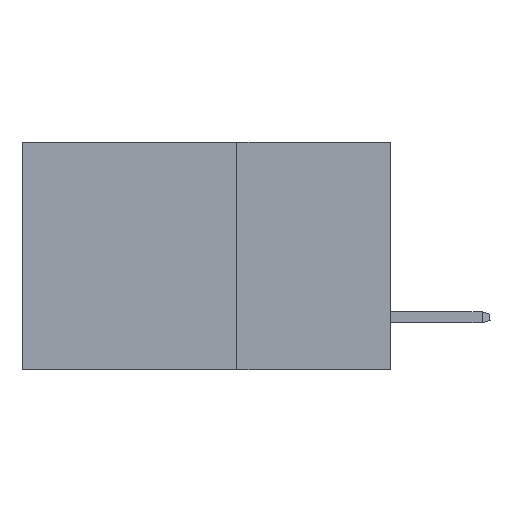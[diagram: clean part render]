
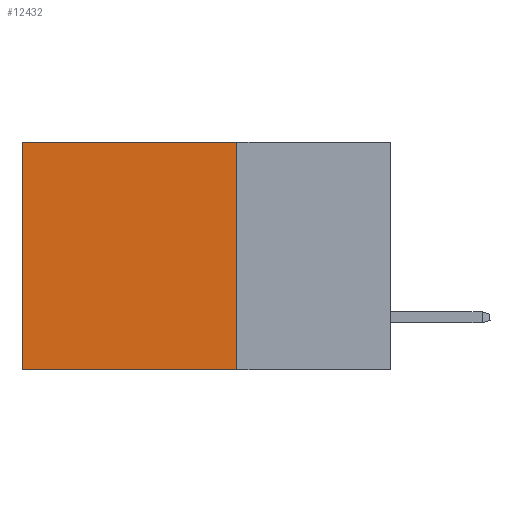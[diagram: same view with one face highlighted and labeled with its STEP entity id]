
A CAD part, left-side view. The second image highlights one B-rep face of the part: STEP entity #12432.
In plain terms, the highlighted planar face has unit normal (-1, 0, 0).
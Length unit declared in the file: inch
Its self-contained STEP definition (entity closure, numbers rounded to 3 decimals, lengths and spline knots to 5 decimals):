
#619 = VECTOR ( 'NONE', #3637, 39.37008 ) ;
#635 = CARTESIAN_POINT ( 'NONE',  ( 0.2875, 0.6, 0. ) ) ;
#852 = DIRECTION ( 'NONE',  ( 0., 0., -1. ) ) ;
#1284 = LINE ( 'NONE', #6132, #2892 ) ;
#1325 = FACE_OUTER_BOUND ( 'NONE', #2107, .T. ) ;
#1583 = CARTESIAN_POINT ( 'NONE',  ( 0.2875, 0.6, 0. ) ) ;
#1838 = DIRECTION ( 'NONE',  ( 0., 0., -1. ) ) ;
#2071 = CARTESIAN_POINT ( 'NONE',  ( 0.2875, 0.25, 0. ) ) ;
#2107 = EDGE_LOOP ( 'NONE', ( #2373, #11663, #14839, #8816 ) ) ;
#2158 = CARTESIAN_POINT ( 'NONE',  ( 0.2875, 0.25, 0. ) ) ;
#2218 = LINE ( 'NONE', #635, #11251 ) ;
#2373 = ORIENTED_EDGE ( 'NONE', *, *, #4997, .T. ) ;
#2892 = VECTOR ( 'NONE', #14164, 39.37008 ) ;
#3637 = DIRECTION ( 'NONE',  ( 0., 1., 0. ) ) ;
#3742 = CARTESIAN_POINT ( 'NONE',  ( 0.2875, 0.25, -0.37 ) ) ;
#4443 = LINE ( 'NONE', #2158, #14905 ) ;
#4629 = VERTEX_POINT ( 'NONE', #9192 ) ;
#4647 = AXIS2_PLACEMENT_3D ( 'NONE', #5303, #6486, #1838 ) ;
#4997 = EDGE_CURVE ( 'NONE', #5737, #4629, #2218, .T. ) ;
#5303 = CARTESIAN_POINT ( 'NONE',  ( 0.2875, 0.25, 0. ) ) ;
#5737 = VERTEX_POINT ( 'NONE', #1583 ) ;
#6132 = CARTESIAN_POINT ( 'NONE',  ( 0.2875, 0.25, 0. ) ) ;
#6486 = DIRECTION ( 'NONE',  ( 1., 0., 0. ) ) ;
#6976 = VERTEX_POINT ( 'NONE', #2071 ) ;
#8618 = LINE ( 'NONE', #3742, #619 ) ;
#8816 = ORIENTED_EDGE ( 'NONE', *, *, #12100, .T. ) ;
#8825 = CARTESIAN_POINT ( 'NONE',  ( 0.2875, 0.25, -0.37 ) ) ;
#8883 = VERTEX_POINT ( 'NONE', #8825 ) ;
#9192 = CARTESIAN_POINT ( 'NONE',  ( 0.2875, 0.6, -0.37 ) ) ;
#11073 = EDGE_CURVE ( 'NONE', #8883, #4629, #8618, .T. ) ;
#11251 = VECTOR ( 'NONE', #852, 39.37008 ) ;
#11357 = DIRECTION ( 'NONE',  ( 0., 1., 0. ) ) ;
#11663 = ORIENTED_EDGE ( 'NONE', *, *, #11073, .F. ) ;
#12100 = EDGE_CURVE ( 'NONE', #6976, #5737, #4443, .T. ) ;
#12196 = PLANE ( 'NONE',  #4647 ) ;
#12432 = ADVANCED_FACE ( 'NONE', ( #1325 ), #12196, .F. ) ;
#14164 = DIRECTION ( 'NONE',  ( 0., 0., -1. ) ) ;
#14431 = EDGE_CURVE ( 'NONE', #6976, #8883, #1284, .T. ) ;
#14839 = ORIENTED_EDGE ( 'NONE', *, *, #14431, .F. ) ;
#14905 = VECTOR ( 'NONE', #11357, 39.37008 ) ;
